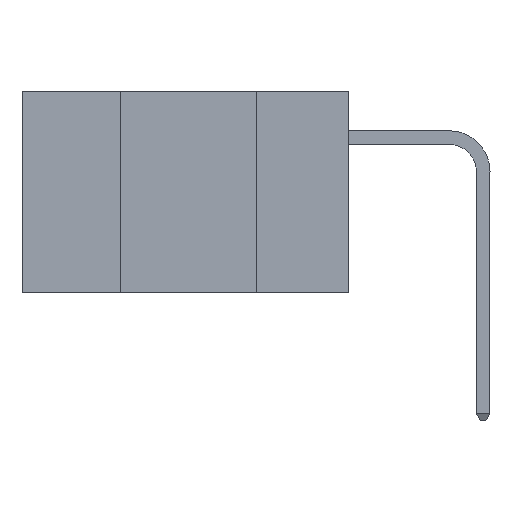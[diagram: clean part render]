
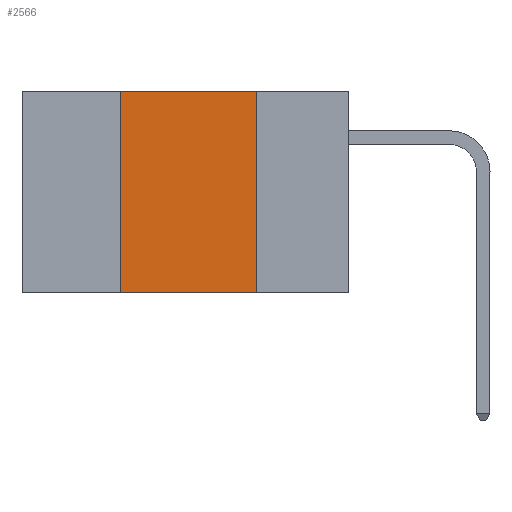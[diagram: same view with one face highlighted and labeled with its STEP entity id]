
A CAD part, left-side view. The second image highlights one B-rep face of the part: STEP entity #2566.
In plain terms, the highlighted planar face has unit normal (-1, 0, 0).
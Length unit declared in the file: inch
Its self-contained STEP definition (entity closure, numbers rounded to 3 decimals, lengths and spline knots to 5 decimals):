
#251 = CARTESIAN_POINT ( 'NONE',  ( 0., 0.6, 0. ) ) ;
#516 = DIRECTION ( 'NONE',  ( 0., -1., 0. ) ) ;
#724 = ORIENTED_EDGE ( 'NONE', *, *, #1409, .F. ) ;
#1134 = EDGE_CURVE ( 'NONE', #14788, #9017, #14292, .T. ) ;
#1409 = EDGE_CURVE ( 'NONE', #15101, #17096, #10409, .T. ) ;
#1946 = CARTESIAN_POINT ( 'NONE',  ( 0., 0.6, 0. ) ) ;
#2393 = CARTESIAN_POINT ( 'NONE',  ( 0., 0.17, 0. ) ) ;
#2566 = ADVANCED_FACE ( 'NONE', ( #2799 ), #7649, .F. ) ;
#2799 = FACE_OUTER_BOUND ( 'NONE', #5937, .T. ) ;
#2814 = VECTOR ( 'NONE', #6843, 39.37008 ) ;
#3019 = CARTESIAN_POINT ( 'NONE',  ( 0., 0.42, -0.37 ) ) ;
#4033 = VECTOR ( 'NONE', #516, 39.37008 ) ;
#4336 = DIRECTION ( 'NONE',  ( 0., 0., -1. ) ) ;
#5937 = EDGE_LOOP ( 'NONE', ( #6877, #13314, #724, #13750 ) ) ;
#6843 = DIRECTION ( 'NONE',  ( 0., 0., 1. ) ) ;
#6877 = ORIENTED_EDGE ( 'NONE', *, *, #1134, .F. ) ;
#7428 = DIRECTION ( 'NONE',  ( 1., 0., 0. ) ) ;
#7508 = CARTESIAN_POINT ( 'NONE',  ( 0., 0.42, 0. ) ) ;
#7649 = PLANE ( 'NONE',  #11243 ) ;
#7722 = EDGE_CURVE ( 'NONE', #15101, #9017, #14423, .T. ) ;
#7976 = CARTESIAN_POINT ( 'NONE',  ( 0., 0.17, 0. ) ) ;
#8256 = LINE ( 'NONE', #1946, #4033 ) ;
#9017 = VERTEX_POINT ( 'NONE', #15738 ) ;
#9892 = VECTOR ( 'NONE', #15634, 39.37008 ) ;
#10317 = EDGE_CURVE ( 'NONE', #17096, #14788, #8256, .T. ) ;
#10409 = LINE ( 'NONE', #16614, #2814 ) ;
#11243 = AXIS2_PLACEMENT_3D ( 'NONE', #251, #7428, #12721 ) ;
#12721 = DIRECTION ( 'NONE',  ( 0., 0., -1. ) ) ;
#13314 = ORIENTED_EDGE ( 'NONE', *, *, #10317, .F. ) ;
#13750 = ORIENTED_EDGE ( 'NONE', *, *, #7722, .T. ) ;
#14268 = CARTESIAN_POINT ( 'NONE',  ( 0., 0.6, -0.37 ) ) ;
#14292 = LINE ( 'NONE', #2393, #17482 ) ;
#14423 = LINE ( 'NONE', #14268, #9892 ) ;
#14788 = VERTEX_POINT ( 'NONE', #7976 ) ;
#15101 = VERTEX_POINT ( 'NONE', #3019 ) ;
#15634 = DIRECTION ( 'NONE',  ( 0., -1., 0. ) ) ;
#15738 = CARTESIAN_POINT ( 'NONE',  ( 0., 0.17, -0.37 ) ) ;
#16614 = CARTESIAN_POINT ( 'NONE',  ( 0., 0.42, 0. ) ) ;
#17096 = VERTEX_POINT ( 'NONE', #7508 ) ;
#17482 = VECTOR ( 'NONE', #4336, 39.37008 ) ;
